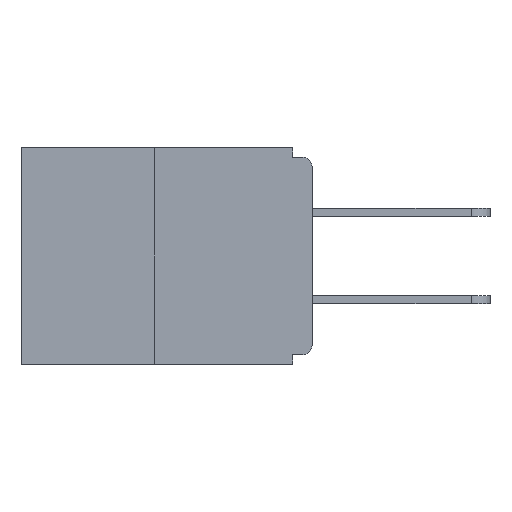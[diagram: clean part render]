
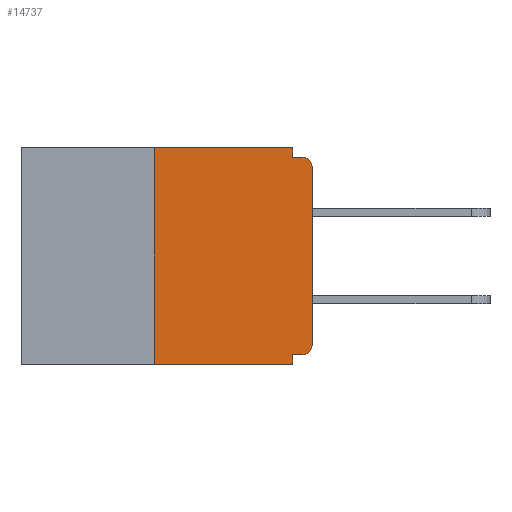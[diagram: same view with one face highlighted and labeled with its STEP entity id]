
A CAD part, left-side view. The second image highlights one B-rep face of the part: STEP entity #14737.
In plain terms, the highlighted planar face has unit normal (-1, 0, 0).
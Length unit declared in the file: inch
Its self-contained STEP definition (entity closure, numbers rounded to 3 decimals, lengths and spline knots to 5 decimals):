
#210 = LINE ( 'NONE', #376, #17447 ) ;
#257 = ORIENTED_EDGE ( 'NONE', *, *, #2342, .T. ) ;
#376 = CARTESIAN_POINT ( 'NONE',  ( 0., 0.25, 0. ) ) ;
#571 = VERTEX_POINT ( 'NONE', #23208 ) ;
#696 = VECTOR ( 'NONE', #27594, 39.37008 ) ;
#1227 = FACE_OUTER_BOUND ( 'NONE', #12851, .T. ) ;
#1285 = VECTOR ( 'NONE', #13900, 39.37008 ) ;
#1369 = CARTESIAN_POINT ( 'NONE',  ( 0., 0.46, 0. ) ) ;
#1388 = CARTESIAN_POINT ( 'NONE',  ( 0., 0.031, -0.328 ) ) ;
#1470 = DIRECTION ( 'NONE',  ( -1., 0., 0. ) ) ;
#1506 = VERTEX_POINT ( 'NONE', #27923 ) ;
#2342 = EDGE_CURVE ( 'NONE', #571, #21760, #6658, .T. ) ;
#2437 = ORIENTED_EDGE ( 'NONE', *, *, #23931, .F. ) ;
#2612 = ORIENTED_EDGE ( 'NONE', *, *, #14193, .F. ) ;
#2710 = ORIENTED_EDGE ( 'NONE', *, *, #5350, .F. ) ;
#2815 = VERTEX_POINT ( 'NONE', #13791 ) ;
#3328 = CARTESIAN_POINT ( 'NONE',  ( 0., 0.015, -0.015 ) ) ;
#3636 = VERTEX_POINT ( 'NONE', #28409 ) ;
#3904 = VERTEX_POINT ( 'NONE', #19760 ) ;
#3959 = AXIS2_PLACEMENT_3D ( 'NONE', #28163, #14877, #5652 ) ;
#4056 = EDGE_CURVE ( 'NONE', #1506, #19757, #17851, .T. ) ;
#4831 = EDGE_CURVE ( 'NONE', #19235, #2815, #29060, .T. ) ;
#4942 = DIRECTION ( 'NONE',  ( -1., 0., 0. ) ) ;
#5082 = VECTOR ( 'NONE', #15104, 39.37008 ) ;
#5107 = VECTOR ( 'NONE', #17699, 39.37008 ) ;
#5350 = EDGE_CURVE ( 'NONE', #25972, #1506, #8612, .T. ) ;
#5517 = ORIENTED_EDGE ( 'NONE', *, *, #21838, .T. ) ;
#5652 = DIRECTION ( 'NONE',  ( 0., 0., -1. ) ) ;
#6658 = CIRCLE ( 'NONE', #28109, 0.015 ) ;
#7719 = LINE ( 'NONE', #25922, #18290 ) ;
#8334 = DIRECTION ( 'NONE',  ( 0., -1., 0. ) ) ;
#8612 = LINE ( 'NONE', #1369, #5082 ) ;
#10164 = DIRECTION ( 'NONE',  ( 0., 0., -1. ) ) ;
#11240 = AXIS2_PLACEMENT_3D ( 'NONE', #21425, #1470, #10164 ) ;
#11572 = CARTESIAN_POINT ( 'NONE',  ( 0., 0.015, -0.03 ) ) ;
#11873 = VECTOR ( 'NONE', #26758, 39.37008 ) ;
#11909 = ORIENTED_EDGE ( 'NONE', *, *, #14521, .T. ) ;
#12424 = PLANE ( 'NONE',  #3959 ) ;
#12539 = CARTESIAN_POINT ( 'NONE',  ( 0., 0.031, -0.343 ) ) ;
#12851 = EDGE_LOOP ( 'NONE', ( #2710, #2437, #5517, #20846, #23336, #23853, #11909, #257, #2612, #23781 ) ) ;
#13027 = VERTEX_POINT ( 'NONE', #18964 ) ;
#13791 = CARTESIAN_POINT ( 'NONE',  ( 0., 0.031, -0.343 ) ) ;
#13900 = DIRECTION ( 'NONE',  ( 0., -1., 0. ) ) ;
#14193 = EDGE_CURVE ( 'NONE', #19757, #21760, #29086, .T. ) ;
#14521 = EDGE_CURVE ( 'NONE', #13027, #571, #23060, .T. ) ;
#14737 = ADVANCED_FACE ( 'NONE', ( #1227 ), #12424, .F. ) ;
#14877 = DIRECTION ( 'NONE',  ( 1., 0., 0. ) ) ;
#15104 = DIRECTION ( 'NONE',  ( 0., -1., 0. ) ) ;
#15751 = CARTESIAN_POINT ( 'NONE',  ( 0., 0., -0.015 ) ) ;
#17447 = VECTOR ( 'NONE', #22991, 39.37008 ) ;
#17699 = DIRECTION ( 'NONE',  ( 0., 0., 1. ) ) ;
#17851 = LINE ( 'NONE', #22048, #11873 ) ;
#17889 = EDGE_CURVE ( 'NONE', #3636, #19235, #26006, .T. ) ;
#18290 = VECTOR ( 'NONE', #8334, 39.37008 ) ;
#18483 = VECTOR ( 'NONE', #19031, 39.37008 ) ;
#18964 = CARTESIAN_POINT ( 'NONE',  ( 0., 0., -0.313 ) ) ;
#19031 = DIRECTION ( 'NONE',  ( 0., 0., -1. ) ) ;
#19235 = VERTEX_POINT ( 'NONE', #1388 ) ;
#19757 = VERTEX_POINT ( 'NONE', #25637 ) ;
#19760 = CARTESIAN_POINT ( 'NONE',  ( 0., 0.25, -0.343 ) ) ;
#20846 = ORIENTED_EDGE ( 'NONE', *, *, #4831, .F. ) ;
#21425 = CARTESIAN_POINT ( 'NONE',  ( 0., 0.015, -0.313 ) ) ;
#21760 = VERTEX_POINT ( 'NONE', #3328 ) ;
#21786 = EDGE_CURVE ( 'NONE', #3636, #13027, #23560, .T. ) ;
#21838 = EDGE_CURVE ( 'NONE', #3904, #2815, #7719, .T. ) ;
#21843 = CARTESIAN_POINT ( 'NONE',  ( 0., 0., 0. ) ) ;
#22048 = CARTESIAN_POINT ( 'NONE',  ( 0., 0.031, 0. ) ) ;
#22991 = DIRECTION ( 'NONE',  ( 0., 0., 1. ) ) ;
#23060 = LINE ( 'NONE', #21843, #5107 ) ;
#23208 = CARTESIAN_POINT ( 'NONE',  ( 0., 0., -0.03 ) ) ;
#23336 = ORIENTED_EDGE ( 'NONE', *, *, #17889, .F. ) ;
#23560 = CIRCLE ( 'NONE', #11240, 0.015 ) ;
#23781 = ORIENTED_EDGE ( 'NONE', *, *, #4056, .F. ) ;
#23853 = ORIENTED_EDGE ( 'NONE', *, *, #21786, .T. ) ;
#23931 = EDGE_CURVE ( 'NONE', #3904, #25972, #210, .T. ) ;
#25213 = CARTESIAN_POINT ( 'NONE',  ( 0., 0.25, 0. ) ) ;
#25524 = CARTESIAN_POINT ( 'NONE',  ( 0., 0., -0.328 ) ) ;
#25637 = CARTESIAN_POINT ( 'NONE',  ( 0., 0.031, -0.015 ) ) ;
#25922 = CARTESIAN_POINT ( 'NONE',  ( 0., 0.46, -0.343 ) ) ;
#25972 = VERTEX_POINT ( 'NONE', #25213 ) ;
#26006 = LINE ( 'NONE', #25524, #696 ) ;
#26758 = DIRECTION ( 'NONE',  ( 0., 0., -1. ) ) ;
#27365 = DIRECTION ( 'NONE',  ( 0., 0., -1. ) ) ;
#27594 = DIRECTION ( 'NONE',  ( 0., 1., 0. ) ) ;
#27923 = CARTESIAN_POINT ( 'NONE',  ( 0., 0.031, 0. ) ) ;
#28109 = AXIS2_PLACEMENT_3D ( 'NONE', #11572, #4942, #27365 ) ;
#28163 = CARTESIAN_POINT ( 'NONE',  ( 0., 0.46, 0. ) ) ;
#28409 = CARTESIAN_POINT ( 'NONE',  ( 0., 0.015, -0.328 ) ) ;
#29060 = LINE ( 'NONE', #12539, #18483 ) ;
#29086 = LINE ( 'NONE', #15751, #1285 ) ;
